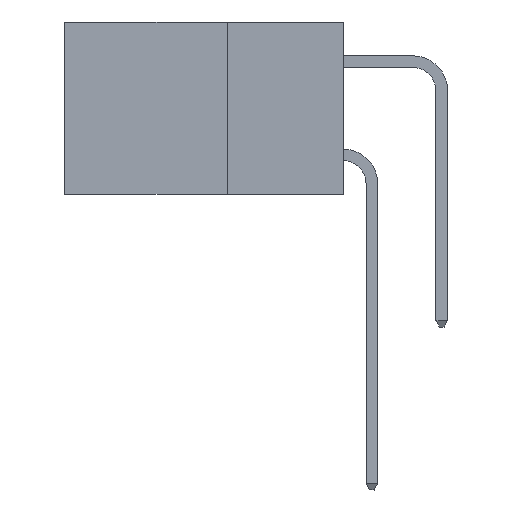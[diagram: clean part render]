
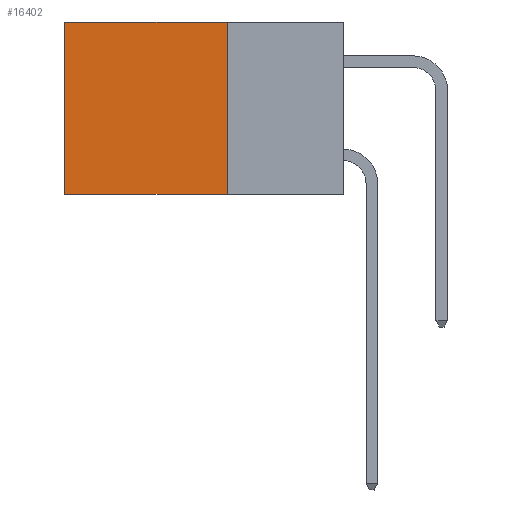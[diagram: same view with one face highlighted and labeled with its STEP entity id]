
A CAD part, left-side view. The second image highlights one B-rep face of the part: STEP entity #16402.
In plain terms, the highlighted planar face has unit normal (-1, 0, 0).
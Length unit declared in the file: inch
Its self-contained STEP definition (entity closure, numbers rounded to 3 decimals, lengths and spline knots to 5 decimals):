
#1280 = ORIENTED_EDGE ( 'NONE', *, *, #1471, .F. ) ;
#1462 = CARTESIAN_POINT ( 'NONE',  ( 0.298, 0.25, 0. ) ) ;
#1471 = EDGE_CURVE ( 'NONE', #3413, #15719, #10524, .T. ) ;
#1491 = VERTEX_POINT ( 'NONE', #1462 ) ;
#1606 = DIRECTION ( 'NONE',  ( 0., 1., 0. ) ) ;
#2383 = PLANE ( 'NONE',  #15082 ) ;
#2620 = EDGE_CURVE ( 'NONE', #1491, #6959, #15789, .T. ) ;
#3413 = VERTEX_POINT ( 'NONE', #5863 ) ;
#4746 = DIRECTION ( 'NONE',  ( 0., 0., -1. ) ) ;
#5648 = VECTOR ( 'NONE', #14521, 39.37008 ) ;
#5863 = CARTESIAN_POINT ( 'NONE',  ( 0.298, 0.25, -0.37 ) ) ;
#5876 = EDGE_CURVE ( 'NONE', #1491, #3413, #14401, .T. ) ;
#5911 = ORIENTED_EDGE ( 'NONE', *, *, #2620, .T. ) ;
#6401 = DIRECTION ( 'NONE',  ( 1., 0., 0. ) ) ;
#6826 = CARTESIAN_POINT ( 'NONE',  ( 0.298, 0.25, 0. ) ) ;
#6959 = VERTEX_POINT ( 'NONE', #14247 ) ;
#8040 = CARTESIAN_POINT ( 'NONE',  ( 0.298, 0.25, -0.37 ) ) ;
#8705 = EDGE_LOOP ( 'NONE', ( #16493, #1280, #16131, #5911 ) ) ;
#10524 = LINE ( 'NONE', #8040, #5648 ) ;
#10603 = EDGE_CURVE ( 'NONE', #6959, #15719, #11754, .T. ) ;
#11754 = LINE ( 'NONE', #11870, #16901 ) ;
#11870 = CARTESIAN_POINT ( 'NONE',  ( 0.298, 0.6, 0. ) ) ;
#12541 = VECTOR ( 'NONE', #4746, 39.37008 ) ;
#12799 = DIRECTION ( 'NONE',  ( 0., 0., -1. ) ) ;
#12885 = CARTESIAN_POINT ( 'NONE',  ( 0.298, 0.6, -0.37 ) ) ;
#13244 = DIRECTION ( 'NONE',  ( 0., 0., -1. ) ) ;
#14168 = CARTESIAN_POINT ( 'NONE',  ( 0.298, 0.25, 0. ) ) ;
#14247 = CARTESIAN_POINT ( 'NONE',  ( 0.298, 0.6, 0. ) ) ;
#14401 = LINE ( 'NONE', #14942, #12541 ) ;
#14521 = DIRECTION ( 'NONE',  ( 0., 1., 0. ) ) ;
#14942 = CARTESIAN_POINT ( 'NONE',  ( 0.298, 0.25, 0. ) ) ;
#15082 = AXIS2_PLACEMENT_3D ( 'NONE', #14168, #6401, #12799 ) ;
#15181 = VECTOR ( 'NONE', #1606, 39.37008 ) ;
#15588 = FACE_OUTER_BOUND ( 'NONE', #8705, .T. ) ;
#15719 = VERTEX_POINT ( 'NONE', #12885 ) ;
#15789 = LINE ( 'NONE', #6826, #15181 ) ;
#16131 = ORIENTED_EDGE ( 'NONE', *, *, #5876, .F. ) ;
#16402 = ADVANCED_FACE ( 'NONE', ( #15588 ), #2383, .F. ) ;
#16493 = ORIENTED_EDGE ( 'NONE', *, *, #10603, .T. ) ;
#16901 = VECTOR ( 'NONE', #13244, 39.37008 ) ;
